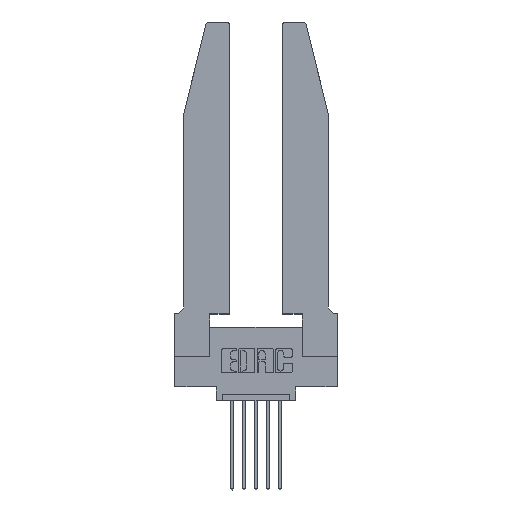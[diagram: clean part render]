
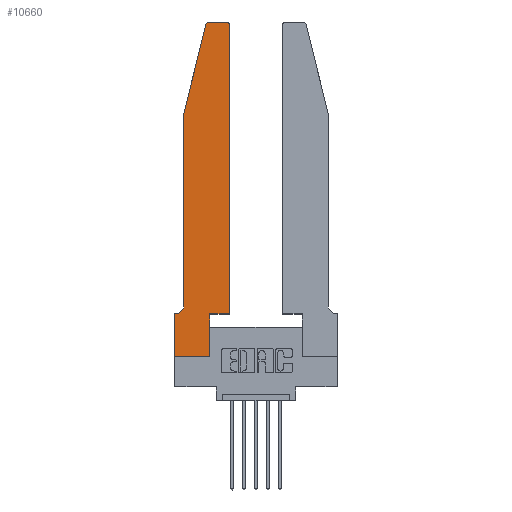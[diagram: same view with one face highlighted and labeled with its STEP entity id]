
A CAD part, top view. The second image highlights one B-rep face of the part: STEP entity #10660.
In plain terms, the highlighted planar face has unit normal (0, 0, 1).
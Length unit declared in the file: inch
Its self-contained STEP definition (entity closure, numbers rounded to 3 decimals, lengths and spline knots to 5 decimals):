
#132 = DIRECTION ( 'NONE',  ( -1., 0., 0. ) ) ;
#279 = EDGE_CURVE ( 'NONE', #12797, #956, #3817, .T. ) ;
#283 = CARTESIAN_POINT ( 'NONE',  ( 0.2865, 0., 0.37 ) ) ;
#333 = VERTEX_POINT ( 'NONE', #11859 ) ;
#382 = CARTESIAN_POINT ( 'NONE',  ( 0., 0., 0.37 ) ) ;
#448 = VERTEX_POINT ( 'NONE', #706 ) ;
#616 = EDGE_CURVE ( 'NONE', #448, #333, #6407, .T. ) ;
#706 = CARTESIAN_POINT ( 'NONE',  ( 0.4205, 2.75, 0.37 ) ) ;
#849 = EDGE_LOOP ( 'NONE', ( #6571, #7237, #5681, #11927, #13019, #9524, #7402, #11383, #7284, #4234, #9406, #8234 ) ) ;
#956 = VERTEX_POINT ( 'NONE', #2785 ) ;
#1102 = CARTESIAN_POINT ( 'NONE',  ( 0.0055, 0.42, 0.37 ) ) ;
#1279 = EDGE_CURVE ( 'NONE', #8808, #448, #4117, .T. ) ;
#1308 = VECTOR ( 'NONE', #1973, 39.37008 ) ;
#1430 = LINE ( 'NONE', #2489, #12630 ) ;
#1594 = CARTESIAN_POINT ( 'NONE',  ( 0.2605, 2.75, 0.37 ) ) ;
#1712 = CARTESIAN_POINT ( 'NONE',  ( 0.284, 2.72, 0.37 ) ) ;
#1736 = CARTESIAN_POINT ( 'NONE',  ( 0., 0.35, 0.37 ) ) ;
#1850 = AXIS2_PLACEMENT_3D ( 'NONE', #1712, #12323, #10272 ) ;
#1879 = VECTOR ( 'NONE', #13323, 39.37008 ) ;
#1973 = DIRECTION ( 'NONE',  ( 0., 1., 0. ) ) ;
#2096 = EDGE_CURVE ( 'NONE', #6358, #12797, #7887, .T. ) ;
#2279 = LINE ( 'NONE', #13165, #8021 ) ;
#2374 = DIRECTION ( 'NONE',  ( 0., -1., 0. ) ) ;
#2489 = CARTESIAN_POINT ( 'NONE',  ( 0., 0., 0.37 ) ) ;
#2500 = VECTOR ( 'NONE', #6329, 39.37008 ) ;
#2571 = LINE ( 'NONE', #12978, #11473 ) ;
#2724 = VERTEX_POINT ( 'NONE', #6760 ) ;
#2785 = CARTESIAN_POINT ( 'NONE',  ( 0.4505, 0.35, 0.37 ) ) ;
#2820 = AXIS2_PLACEMENT_3D ( 'NONE', #9853, #10967, #5698 ) ;
#2918 = CARTESIAN_POINT ( 'NONE',  ( 0.0755, 2., 0.37 ) ) ;
#3187 = VERTEX_POINT ( 'NONE', #9666 ) ;
#3344 = EDGE_CURVE ( 'NONE', #9840, #12396, #2279, .T. ) ;
#3644 = VECTOR ( 'NONE', #12172, 39.37008 ) ;
#3817 = LINE ( 'NONE', #11813, #2500 ) ;
#3936 = DIRECTION ( 'NONE',  ( 0., 0., 1. ) ) ;
#4117 = CIRCLE ( 'NONE', #2820, 0.03 ) ;
#4234 = ORIENTED_EDGE ( 'NONE', *, *, #279, .T. ) ;
#4398 = CARTESIAN_POINT ( 'NONE',  ( 0.0055, 0.35, 0.37 ) ) ;
#4419 = CIRCLE ( 'NONE', #1850, 0.03 ) ;
#4503 = DIRECTION ( 'NONE',  ( -0.239, -0.971, 0. ) ) ;
#4633 = LINE ( 'NONE', #2918, #1879 ) ;
#4713 = EDGE_CURVE ( 'NONE', #9912, #3187, #2571, .T. ) ;
#5176 = LINE ( 'NONE', #382, #6002 ) ;
#5313 = EDGE_CURVE ( 'NONE', #12396, #9943, #5176, .T. ) ;
#5377 = DIRECTION ( 'NONE',  ( 0., 0., -1. ) ) ;
#5681 = ORIENTED_EDGE ( 'NONE', *, *, #4713, .T. ) ;
#5698 = DIRECTION ( 'NONE',  ( 1., 0., 0. ) ) ;
#6002 = VECTOR ( 'NONE', #2374, 39.37008 ) ;
#6029 = DIRECTION ( 'NONE',  ( 1., 0., 0. ) ) ;
#6076 = CARTESIAN_POINT ( 'NONE',  ( 0.2865, 0.35, 0.37 ) ) ;
#6329 = DIRECTION ( 'NONE',  ( 1., 0., 0. ) ) ;
#6358 = VERTEX_POINT ( 'NONE', #283 ) ;
#6407 = LINE ( 'NONE', #1594, #3644 ) ;
#6571 = ORIENTED_EDGE ( 'NONE', *, *, #616, .T. ) ;
#6717 = LINE ( 'NONE', #10757, #7380 ) ;
#6760 = CARTESIAN_POINT ( 'NONE',  ( 0.0755, 0.42, 0.37 ) ) ;
#7092 = AXIS2_PLACEMENT_3D ( 'NONE', #1102, #5377, #132 ) ;
#7103 = CIRCLE ( 'NONE', #7092, 0.07 ) ;
#7237 = ORIENTED_EDGE ( 'NONE', *, *, #12335, .T. ) ;
#7284 = ORIENTED_EDGE ( 'NONE', *, *, #2096, .T. ) ;
#7380 = VECTOR ( 'NONE', #11688, 39.37008 ) ;
#7402 = ORIENTED_EDGE ( 'NONE', *, *, #5313, .T. ) ;
#7826 = CARTESIAN_POINT ( 'NONE',  ( 0.2865, 0.35, 0.37 ) ) ;
#7887 = LINE ( 'NONE', #6076, #1308 ) ;
#7929 = EDGE_CURVE ( 'NONE', #9943, #6358, #1430, .T. ) ;
#8021 = VECTOR ( 'NONE', #12125, 39.37008 ) ;
#8117 = PLANE ( 'NONE',  #12582 ) ;
#8234 = ORIENTED_EDGE ( 'NONE', *, *, #1279, .T. ) ;
#8808 = VERTEX_POINT ( 'NONE', #10391 ) ;
#9406 = ORIENTED_EDGE ( 'NONE', *, *, #11974, .T. ) ;
#9524 = ORIENTED_EDGE ( 'NONE', *, *, #3344, .T. ) ;
#9666 = CARTESIAN_POINT ( 'NONE',  ( 0.0755, 2., 0.37 ) ) ;
#9840 = VERTEX_POINT ( 'NONE', #4398 ) ;
#9853 = CARTESIAN_POINT ( 'NONE',  ( 0.4205, 2.72, 0.37 ) ) ;
#9912 = VERTEX_POINT ( 'NONE', #12072 ) ;
#9943 = VERTEX_POINT ( 'NONE', #13056 ) ;
#10272 = DIRECTION ( 'NONE',  ( 1., 0., 0. ) ) ;
#10391 = CARTESIAN_POINT ( 'NONE',  ( 0.4505, 2.72, 0.37 ) ) ;
#10660 = ADVANCED_FACE ( 'NONE', ( #13043 ), #8117, .T. ) ;
#10680 = EDGE_CURVE ( 'NONE', #3187, #2724, #4633, .T. ) ;
#10757 = CARTESIAN_POINT ( 'NONE',  ( 0.4505, 0.35, 0.37 ) ) ;
#10879 = EDGE_CURVE ( 'NONE', #2724, #9840, #7103, .T. ) ;
#10967 = DIRECTION ( 'NONE',  ( 0., 0., 1. ) ) ;
#11383 = ORIENTED_EDGE ( 'NONE', *, *, #7929, .T. ) ;
#11473 = VECTOR ( 'NONE', #4503, 39.37008 ) ;
#11688 = DIRECTION ( 'NONE',  ( 0., 1., 0. ) ) ;
#11800 = DIRECTION ( 'NONE',  ( 1., 0., 0. ) ) ;
#11813 = CARTESIAN_POINT ( 'NONE',  ( 0.4505, 0.35, 0.37 ) ) ;
#11859 = CARTESIAN_POINT ( 'NONE',  ( 0.284, 2.75, 0.37 ) ) ;
#11927 = ORIENTED_EDGE ( 'NONE', *, *, #10680, .T. ) ;
#11974 = EDGE_CURVE ( 'NONE', #956, #8808, #6717, .T. ) ;
#12072 = CARTESIAN_POINT ( 'NONE',  ( 0.25487, 2.72718, 0.37 ) ) ;
#12125 = DIRECTION ( 'NONE',  ( -1., 0., 0. ) ) ;
#12172 = DIRECTION ( 'NONE',  ( -1., 0., 0. ) ) ;
#12323 = DIRECTION ( 'NONE',  ( 0., 0., 1. ) ) ;
#12335 = EDGE_CURVE ( 'NONE', #333, #9912, #4419, .T. ) ;
#12396 = VERTEX_POINT ( 'NONE', #13434 ) ;
#12582 = AXIS2_PLACEMENT_3D ( 'NONE', #1736, #3936, #6029 ) ;
#12630 = VECTOR ( 'NONE', #11800, 39.37008 ) ;
#12797 = VERTEX_POINT ( 'NONE', #7826 ) ;
#12978 = CARTESIAN_POINT ( 'NONE',  ( 0.0755, 2., 0.37 ) ) ;
#13019 = ORIENTED_EDGE ( 'NONE', *, *, #10879, .T. ) ;
#13043 = FACE_OUTER_BOUND ( 'NONE', #849, .T. ) ;
#13056 = CARTESIAN_POINT ( 'NONE',  ( 0., 0., 0.37 ) ) ;
#13165 = CARTESIAN_POINT ( 'NONE',  ( 0.0755, 0.35, 0.37 ) ) ;
#13323 = DIRECTION ( 'NONE',  ( 0., -1., 0. ) ) ;
#13434 = CARTESIAN_POINT ( 'NONE',  ( 0., 0.35, 0.37 ) ) ;
